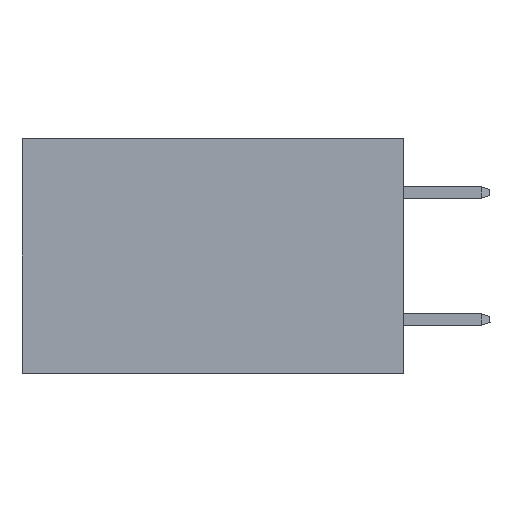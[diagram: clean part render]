
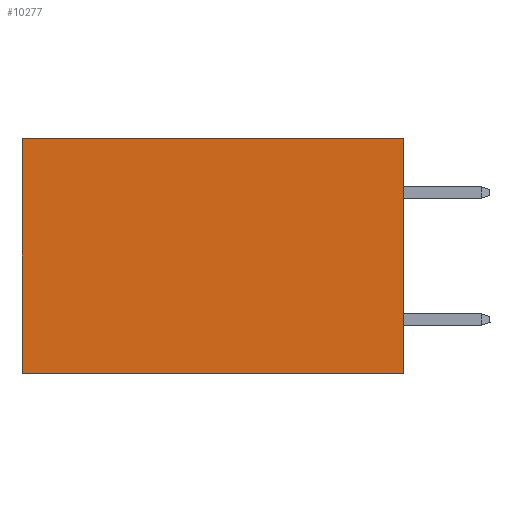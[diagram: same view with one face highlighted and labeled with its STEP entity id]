
A CAD part, left-side view. The second image highlights one B-rep face of the part: STEP entity #10277.
In plain terms, the highlighted planar face has unit normal (-1, 0, 0).
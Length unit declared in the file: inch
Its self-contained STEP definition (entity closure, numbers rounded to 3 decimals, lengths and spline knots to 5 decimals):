
#320 = CARTESIAN_POINT ( 'NONE',  ( 0.2875, 0., 0. ) ) ;
#860 = DIRECTION ( 'NONE',  ( 0., 0., -1. ) ) ;
#1091 = LINE ( 'NONE', #5113, #13864 ) ;
#1740 = ORIENTED_EDGE ( 'NONE', *, *, #4918, .T. ) ;
#2061 = EDGE_CURVE ( 'NONE', #17049, #4245, #16737, .T. ) ;
#2360 = LINE ( 'NONE', #16229, #14947 ) ;
#3764 = ORIENTED_EDGE ( 'NONE', *, *, #9479, .F. ) ;
#4245 = VERTEX_POINT ( 'NONE', #14505 ) ;
#4918 = EDGE_CURVE ( 'NONE', #17049, #15628, #1091, .T. ) ;
#4951 = CARTESIAN_POINT ( 'NONE',  ( 0.2875, 0.6, 0. ) ) ;
#4974 = CARTESIAN_POINT ( 'NONE',  ( 0.2875, 0.6, -0.37 ) ) ;
#5062 = DIRECTION ( 'NONE',  ( 0., 0., -1. ) ) ;
#5113 = CARTESIAN_POINT ( 'NONE',  ( 0.2875, 0., 0. ) ) ;
#5805 = CARTESIAN_POINT ( 'NONE',  ( 0.2875, 0., 0. ) ) ;
#6261 = DIRECTION ( 'NONE',  ( 0., 1., 0. ) ) ;
#6555 = VECTOR ( 'NONE', #860, 39.37008 ) ;
#6893 = EDGE_LOOP ( 'NONE', ( #19835, #3764, #23385, #1740 ) ) ;
#8366 = DIRECTION ( 'NONE',  ( 0., 0., -1. ) ) ;
#9479 = EDGE_CURVE ( 'NONE', #4245, #13955, #2360, .T. ) ;
#10277 = ADVANCED_FACE ( 'NONE', ( #25372 ), #16853, .F. ) ;
#11189 = VECTOR ( 'NONE', #8366, 39.37008 ) ;
#13864 = VECTOR ( 'NONE', #24948, 39.37008 ) ;
#13955 = VERTEX_POINT ( 'NONE', #4974 ) ;
#14505 = CARTESIAN_POINT ( 'NONE',  ( 0.2875, 0., -0.37 ) ) ;
#14749 = CARTESIAN_POINT ( 'NONE',  ( 0.2875, 0.6, 0. ) ) ;
#14947 = VECTOR ( 'NONE', #6261, 39.37008 ) ;
#15628 = VERTEX_POINT ( 'NONE', #4951 ) ;
#16229 = CARTESIAN_POINT ( 'NONE',  ( 0.2875, 0., -0.37 ) ) ;
#16737 = LINE ( 'NONE', #320, #11189 ) ;
#16853 = PLANE ( 'NONE',  #20162 ) ;
#17049 = VERTEX_POINT ( 'NONE', #19584 ) ;
#17685 = EDGE_CURVE ( 'NONE', #15628, #13955, #22505, .T. ) ;
#19584 = CARTESIAN_POINT ( 'NONE',  ( 0.2875, 0., 0. ) ) ;
#19835 = ORIENTED_EDGE ( 'NONE', *, *, #17685, .T. ) ;
#20162 = AXIS2_PLACEMENT_3D ( 'NONE', #5805, #24895, #5062 ) ;
#22505 = LINE ( 'NONE', #14749, #6555 ) ;
#23385 = ORIENTED_EDGE ( 'NONE', *, *, #2061, .F. ) ;
#24895 = DIRECTION ( 'NONE',  ( 1., 0., 0. ) ) ;
#24948 = DIRECTION ( 'NONE',  ( 0., 1., 0. ) ) ;
#25372 = FACE_OUTER_BOUND ( 'NONE', #6893, .T. ) ;
